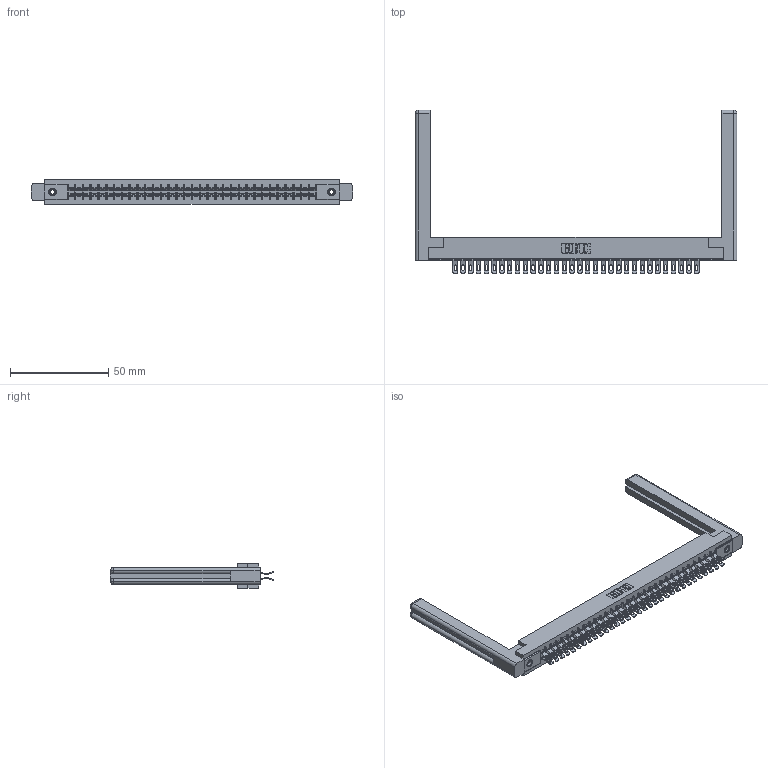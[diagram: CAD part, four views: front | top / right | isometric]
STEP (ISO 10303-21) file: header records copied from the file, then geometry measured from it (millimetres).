
FILE_DESCRIPTION (( 'STEP AP203' ), '1' );
FILE_NAME ('305-064-555-558.STEP', '2019-09-10T02:59:59', ( '' ), ( '' ), 'SwSTEP 2.0', 'SolidWorks 2016', '' );
FILE_SCHEMA (( 'CONFIG_CONTROL_DESIGN' ));
Length unit declared in the file: inch
Products named in the file (5): 305-064-555-558; 345-250-001_345-250-001-102; 305-290-001_555; 307-220-058; 305 Part_.156 Dia
Assembly tree (69 placements, depth 2):
  305-064-555-558
    305 Part_.156 Dia
    305-290-001_555  x64
    345-250-001_345-250-001-102  x2
    307-220-058  x2
Bounding box: 163.42 x 83.06 x 12.7 mm (x, y, z)
Volume: 23891.7 mm3; surface area: 27834.9 mm2
Topology: 69 solids, 69 shells, 4482 faces, 13310 edges, 8688 vertices
Faces by surface type: plane 2200, cylinder 2130, sphere 128, cone 12, torus 12
Entity records: 39122 total; most frequent: CARTESIAN_POINT 6507, ORIENTED_EDGE 6390, DIRECTION 6259, EDGE_CURVE 3195, VECTOR 2543, LINE 2543, VERTEX_POINT 2036, AXIS2_PLACEMENT_3D 1858
